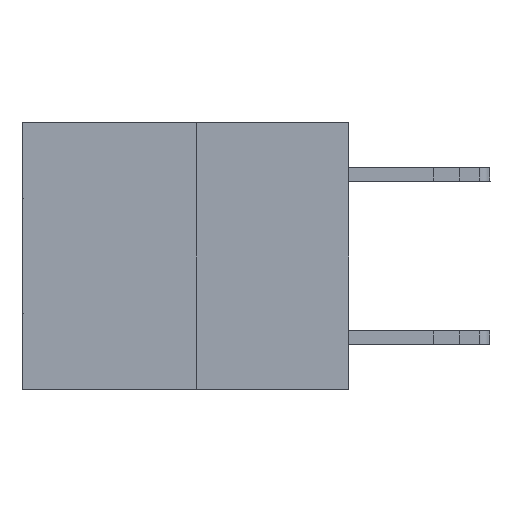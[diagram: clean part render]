
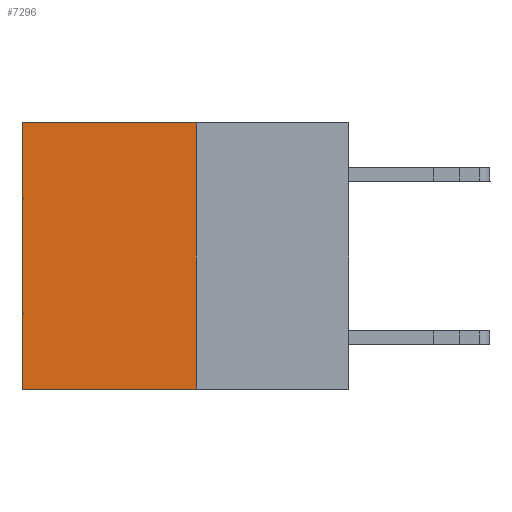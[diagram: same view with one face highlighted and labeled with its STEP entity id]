
A CAD part, left-side view. The second image highlights one B-rep face of the part: STEP entity #7296.
In plain terms, the highlighted planar face has unit normal (-1, 0, 0).
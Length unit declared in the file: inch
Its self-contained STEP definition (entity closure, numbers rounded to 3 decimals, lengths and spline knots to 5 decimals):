
#382 = DIRECTION ( 'NONE',  ( 0., 0., -1. ) ) ;
#491 = CARTESIAN_POINT ( 'NONE',  ( 0.3165, 0.28, -0.49 ) ) ;
#1509 = DIRECTION ( 'NONE',  ( 0., 1., 0. ) ) ;
#3285 = ORIENTED_EDGE ( 'NONE', *, *, #18146, .T. ) ;
#3362 = CARTESIAN_POINT ( 'NONE',  ( 0.3165, 0.28, 0. ) ) ;
#3826 = VECTOR ( 'NONE', #15751, 39.37008 ) ;
#3997 = ORIENTED_EDGE ( 'NONE', *, *, #21497, .F. ) ;
#5234 = CARTESIAN_POINT ( 'NONE',  ( 0.3165, 0.28, -0.49 ) ) ;
#5489 = VECTOR ( 'NONE', #10784, 39.37008 ) ;
#5633 = CARTESIAN_POINT ( 'NONE',  ( 0.3165, 0.28, -0.49 ) ) ;
#5778 = DIRECTION ( 'NONE',  ( 0., 0., -1. ) ) ;
#7296 = ADVANCED_FACE ( 'NONE', ( #15704 ), #12404, .F. ) ;
#10780 = CARTESIAN_POINT ( 'NONE',  ( 0.3165, 0.6, -0.49 ) ) ;
#10784 = DIRECTION ( 'NONE',  ( 0., 1., 0. ) ) ;
#10849 = LINE ( 'NONE', #10780, #3826 ) ;
#11032 = VERTEX_POINT ( 'NONE', #14764 ) ;
#11362 = VERTEX_POINT ( 'NONE', #5234 ) ;
#11762 = LINE ( 'NONE', #5633, #5489 ) ;
#12404 = PLANE ( 'NONE',  #22210 ) ;
#12960 = CARTESIAN_POINT ( 'NONE',  ( 0.3165, 0.6, 0. ) ) ;
#13089 = LINE ( 'NONE', #17485, #16000 ) ;
#13504 = VERTEX_POINT ( 'NONE', #22086 ) ;
#14571 = ORIENTED_EDGE ( 'NONE', *, *, #29387, .T. ) ;
#14764 = CARTESIAN_POINT ( 'NONE',  ( 0.3165, 0.6, -0.49 ) ) ;
#15704 = FACE_OUTER_BOUND ( 'NONE', #23174, .T. ) ;
#15751 = DIRECTION ( 'NONE',  ( 0., 0., -1. ) ) ;
#16000 = VECTOR ( 'NONE', #5778, 39.37008 ) ;
#17107 = LINE ( 'NONE', #3362, #22287 ) ;
#17485 = CARTESIAN_POINT ( 'NONE',  ( 0.3165, 0.28, -0.49 ) ) ;
#18146 = EDGE_CURVE ( 'NONE', #22633, #11032, #10849, .T. ) ;
#19110 = DIRECTION ( 'NONE',  ( 1., 0., 0. ) ) ;
#21497 = EDGE_CURVE ( 'NONE', #11362, #11032, #11762, .T. ) ;
#21844 = ORIENTED_EDGE ( 'NONE', *, *, #29112, .F. ) ;
#22086 = CARTESIAN_POINT ( 'NONE',  ( 0.3165, 0.28, 0. ) ) ;
#22210 = AXIS2_PLACEMENT_3D ( 'NONE', #491, #19110, #382 ) ;
#22287 = VECTOR ( 'NONE', #1509, 39.37008 ) ;
#22633 = VERTEX_POINT ( 'NONE', #12960 ) ;
#23174 = EDGE_LOOP ( 'NONE', ( #3285, #3997, #21844, #14571 ) ) ;
#29112 = EDGE_CURVE ( 'NONE', #13504, #11362, #13089, .T. ) ;
#29387 = EDGE_CURVE ( 'NONE', #13504, #22633, #17107, .T. ) ;
